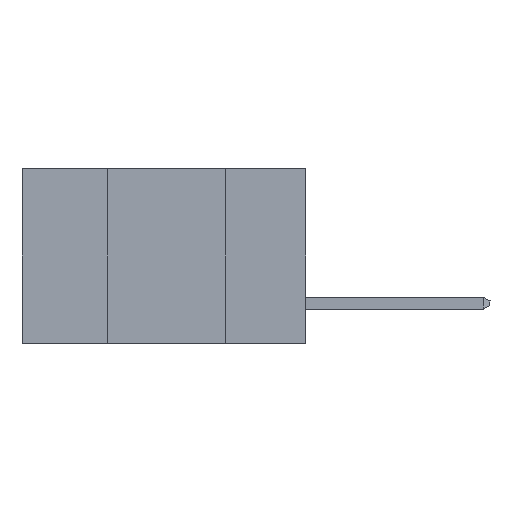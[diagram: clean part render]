
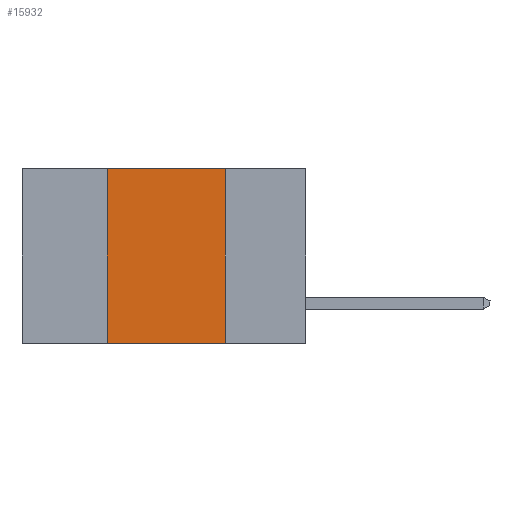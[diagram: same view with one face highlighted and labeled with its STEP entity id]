
A CAD part, left-side view. The second image highlights one B-rep face of the part: STEP entity #15932.
In plain terms, the highlighted planar face has unit normal (-1, 0, 0).
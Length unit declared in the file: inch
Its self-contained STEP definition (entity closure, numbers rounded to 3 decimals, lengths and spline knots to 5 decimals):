
#3257 = EDGE_CURVE ( 'NONE', #22976, #10799, #5898, .T. ) ;
#3377 = LINE ( 'NONE', #24215, #13072 ) ;
#3426 = CARTESIAN_POINT ( 'NONE',  ( 0., 0.6, 0. ) ) ;
#4535 = EDGE_LOOP ( 'NONE', ( #11706, #21548, #23060, #22075 ) ) ;
#4999 = DIRECTION ( 'NONE',  ( 0., 0., -1. ) ) ;
#5738 = EDGE_CURVE ( 'NONE', #22976, #14611, #13159, .T. ) ;
#5898 = LINE ( 'NONE', #21777, #10763 ) ;
#7286 = EDGE_CURVE ( 'NONE', #10799, #18348, #26461, .T. ) ;
#7919 = VECTOR ( 'NONE', #10244, 39.37008 ) ;
#10244 = DIRECTION ( 'NONE',  ( 0., -1., 0. ) ) ;
#10763 = VECTOR ( 'NONE', #26124, 39.37008 ) ;
#10799 = VERTEX_POINT ( 'NONE', #24552 ) ;
#11170 = FACE_OUTER_BOUND ( 'NONE', #4535, .T. ) ;
#11706 = ORIENTED_EDGE ( 'NONE', *, *, #25124, .F. ) ;
#13072 = VECTOR ( 'NONE', #4999, 39.37008 ) ;
#13159 = LINE ( 'NONE', #17939, #16145 ) ;
#13387 = DIRECTION ( 'NONE',  ( 0., -1., 0. ) ) ;
#13825 = AXIS2_PLACEMENT_3D ( 'NONE', #29357, #17314, #17632 ) ;
#14138 = CARTESIAN_POINT ( 'NONE',  ( 0., 0.17, -0.37 ) ) ;
#14611 = VERTEX_POINT ( 'NONE', #14138 ) ;
#15932 = ADVANCED_FACE ( 'NONE', ( #11170 ), #19711, .F. ) ;
#16145 = VECTOR ( 'NONE', #13387, 39.37008 ) ;
#17314 = DIRECTION ( 'NONE',  ( 1., 0., 0. ) ) ;
#17632 = DIRECTION ( 'NONE',  ( 0., 0., -1. ) ) ;
#17939 = CARTESIAN_POINT ( 'NONE',  ( 0., 0.6, -0.37 ) ) ;
#18348 = VERTEX_POINT ( 'NONE', #30628 ) ;
#19711 = PLANE ( 'NONE',  #13825 ) ;
#21548 = ORIENTED_EDGE ( 'NONE', *, *, #7286, .F. ) ;
#21777 = CARTESIAN_POINT ( 'NONE',  ( 0., 0.42, 0. ) ) ;
#22075 = ORIENTED_EDGE ( 'NONE', *, *, #5738, .T. ) ;
#22976 = VERTEX_POINT ( 'NONE', #29129 ) ;
#23060 = ORIENTED_EDGE ( 'NONE', *, *, #3257, .F. ) ;
#24215 = CARTESIAN_POINT ( 'NONE',  ( 0., 0.17, 0. ) ) ;
#24552 = CARTESIAN_POINT ( 'NONE',  ( 0., 0.42, 0. ) ) ;
#25124 = EDGE_CURVE ( 'NONE', #18348, #14611, #3377, .T. ) ;
#26124 = DIRECTION ( 'NONE',  ( 0., 0., 1. ) ) ;
#26461 = LINE ( 'NONE', #3426, #7919 ) ;
#29129 = CARTESIAN_POINT ( 'NONE',  ( 0., 0.42, -0.37 ) ) ;
#29357 = CARTESIAN_POINT ( 'NONE',  ( 0., 0.6, 0. ) ) ;
#30628 = CARTESIAN_POINT ( 'NONE',  ( 0., 0.17, 0. ) ) ;
